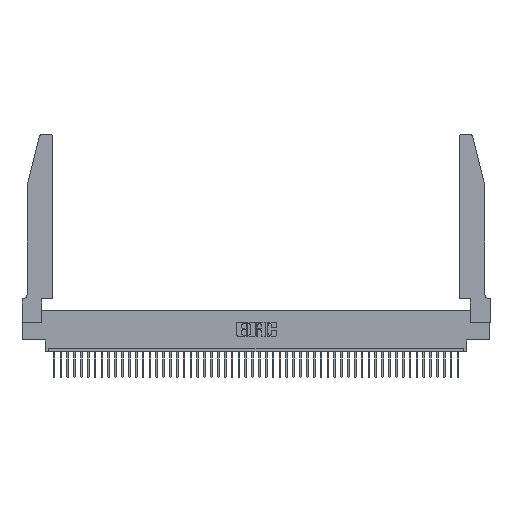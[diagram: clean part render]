
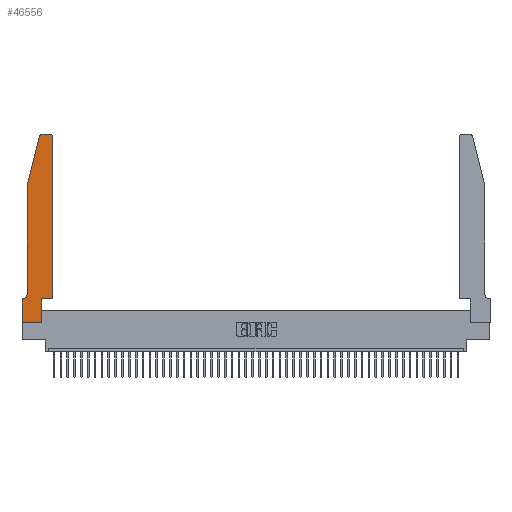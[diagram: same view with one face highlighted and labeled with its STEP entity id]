
A CAD part, top view. The second image highlights one B-rep face of the part: STEP entity #46556.
In plain terms, the highlighted planar face has unit normal (0, 0, 1).
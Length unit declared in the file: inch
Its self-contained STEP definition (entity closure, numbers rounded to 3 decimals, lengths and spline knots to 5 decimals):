
#683 = DIRECTION ( 'NONE',  ( 0., 1., 0. ) ) ;
#1280 = EDGE_LOOP ( 'NONE', ( #1739, #37646, #26872, #36971, #42703, #25595, #14816, #1479, #3994, #7555, #30606, #16357 ) ) ;
#1479 = ORIENTED_EDGE ( 'NONE', *, *, #37676, .T. ) ;
#1739 = ORIENTED_EDGE ( 'NONE', *, *, #34927, .T. ) ;
#2262 = LINE ( 'NONE', #24176, #37366 ) ;
#2815 = DIRECTION ( 'NONE',  ( 0., -1., 0. ) ) ;
#2891 = CARTESIAN_POINT ( 'NONE',  ( 0.0755, 0.42, 0.37 ) ) ;
#3130 = DIRECTION ( 'NONE',  ( 1., 0., 0. ) ) ;
#3139 = CARTESIAN_POINT ( 'NONE',  ( 0.0755, 2., 0.37 ) ) ;
#3725 = CARTESIAN_POINT ( 'NONE',  ( 0.25487, 2.72718, 0.37 ) ) ;
#3811 = EDGE_CURVE ( 'NONE', #37663, #9982, #31243, .T. ) ;
#3994 = ORIENTED_EDGE ( 'NONE', *, *, #32606, .T. ) ;
#4002 = CARTESIAN_POINT ( 'NONE',  ( 0.0055, 0.35, 0.37 ) ) ;
#4797 = VECTOR ( 'NONE', #9925, 39.37008 ) ;
#5273 = LINE ( 'NONE', #45043, #19057 ) ;
#5633 = CARTESIAN_POINT ( 'NONE',  ( 0.4505, 0.35, 0.37 ) ) ;
#5794 = LINE ( 'NONE', #20876, #12665 ) ;
#5851 = EDGE_CURVE ( 'NONE', #29223, #14498, #2262, .T. ) ;
#6450 = VERTEX_POINT ( 'NONE', #15309 ) ;
#7297 = VERTEX_POINT ( 'NONE', #3725 ) ;
#7555 = ORIENTED_EDGE ( 'NONE', *, *, #16457, .T. ) ;
#7649 = VERTEX_POINT ( 'NONE', #30393 ) ;
#8221 = EDGE_CURVE ( 'NONE', #26927, #13217, #12668, .T. ) ;
#8306 = DIRECTION ( 'NONE',  ( 0., 0., 1. ) ) ;
#8960 = CARTESIAN_POINT ( 'NONE',  ( 0.0755, 2., 0.37 ) ) ;
#9444 = VECTOR ( 'NONE', #21039, 39.37008 ) ;
#9925 = DIRECTION ( 'NONE',  ( -0.239, -0.971, 0. ) ) ;
#9982 = VERTEX_POINT ( 'NONE', #30535 ) ;
#11241 = FACE_OUTER_BOUND ( 'NONE', #1280, .T. ) ;
#12665 = VECTOR ( 'NONE', #46744, 39.37008 ) ;
#12668 = LINE ( 'NONE', #3139, #46632 ) ;
#12776 = CARTESIAN_POINT ( 'NONE',  ( 0.4505, 0.35, 0.37 ) ) ;
#13217 = VERTEX_POINT ( 'NONE', #2891 ) ;
#14498 = VERTEX_POINT ( 'NONE', #45339 ) ;
#14816 = ORIENTED_EDGE ( 'NONE', *, *, #40210, .T. ) ;
#15309 = CARTESIAN_POINT ( 'NONE',  ( 0.2865, 0.35, 0.37 ) ) ;
#15660 = DIRECTION ( 'NONE',  ( 0., -1., 0. ) ) ;
#16357 = ORIENTED_EDGE ( 'NONE', *, *, #33684, .T. ) ;
#16457 = EDGE_CURVE ( 'NONE', #6450, #37663, #5794, .T. ) ;
#17316 = CARTESIAN_POINT ( 'NONE',  ( 0.0755, 2., 0.37 ) ) ;
#18420 = DIRECTION ( 'NONE',  ( 1., 0., 0. ) ) ;
#18593 = CARTESIAN_POINT ( 'NONE',  ( 0.2865, 0., 0.37 ) ) ;
#19057 = VECTOR ( 'NONE', #683, 39.37008 ) ;
#19262 = LINE ( 'NONE', #46527, #32524 ) ;
#19546 = VERTEX_POINT ( 'NONE', #18593 ) ;
#19833 = DIRECTION ( 'NONE',  ( -1., 0., 0. ) ) ;
#20710 = VERTEX_POINT ( 'NONE', #25222 ) ;
#20876 = CARTESIAN_POINT ( 'NONE',  ( 0.4505, 0.35, 0.37 ) ) ;
#21039 = DIRECTION ( 'NONE',  ( -1., 0., 0. ) ) ;
#22398 = AXIS2_PLACEMENT_3D ( 'NONE', #28205, #28688, #3130 ) ;
#22547 = LINE ( 'NONE', #17316, #4797 ) ;
#23108 = LINE ( 'NONE', #44593, #45009 ) ;
#23530 = CIRCLE ( 'NONE', #43765, 0.03 ) ;
#24176 = CARTESIAN_POINT ( 'NONE',  ( 0.0755, 0.35, 0.37 ) ) ;
#25222 = CARTESIAN_POINT ( 'NONE',  ( 0., 0., 0.37 ) ) ;
#25595 = ORIENTED_EDGE ( 'NONE', *, *, #5851, .T. ) ;
#25815 = CARTESIAN_POINT ( 'NONE',  ( 0.4205, 2.72, 0.37 ) ) ;
#26767 = CARTESIAN_POINT ( 'NONE',  ( 0.284, 2.72, 0.37 ) ) ;
#26872 = ORIENTED_EDGE ( 'NONE', *, *, #35549, .T. ) ;
#26927 = VERTEX_POINT ( 'NONE', #8960 ) ;
#28205 = CARTESIAN_POINT ( 'NONE',  ( 0., 0.35, 0.37 ) ) ;
#28688 = DIRECTION ( 'NONE',  ( 0., 0., 1. ) ) ;
#28743 = DIRECTION ( 'NONE',  ( 0., 0., 1. ) ) ;
#29223 = VERTEX_POINT ( 'NONE', #4002 ) ;
#30393 = CARTESIAN_POINT ( 'NONE',  ( 0.4205, 2.75, 0.37 ) ) ;
#30535 = CARTESIAN_POINT ( 'NONE',  ( 0.4505, 2.72, 0.37 ) ) ;
#30606 = ORIENTED_EDGE ( 'NONE', *, *, #3811, .T. ) ;
#30744 = VERTEX_POINT ( 'NONE', #34599 ) ;
#31243 = LINE ( 'NONE', #5633, #45607 ) ;
#31320 = LINE ( 'NONE', #38427, #9444 ) ;
#32524 = VECTOR ( 'NONE', #38518, 39.37008 ) ;
#32606 = EDGE_CURVE ( 'NONE', #19546, #6450, #5273, .T. ) ;
#33684 = EDGE_CURVE ( 'NONE', #9982, #7649, #23530, .T. ) ;
#34569 = DIRECTION ( 'NONE',  ( 0., 1., 0. ) ) ;
#34599 = CARTESIAN_POINT ( 'NONE',  ( 0.284, 2.75, 0.37 ) ) ;
#34927 = EDGE_CURVE ( 'NONE', #7649, #30744, #31320, .T. ) ;
#35549 = EDGE_CURVE ( 'NONE', #7297, #26927, #22547, .T. ) ;
#35921 = EDGE_CURVE ( 'NONE', #13217, #29223, #45556, .T. ) ;
#36971 = ORIENTED_EDGE ( 'NONE', *, *, #8221, .T. ) ;
#37366 = VECTOR ( 'NONE', #40913, 39.37008 ) ;
#37646 = ORIENTED_EDGE ( 'NONE', *, *, #46249, .T. ) ;
#37663 = VERTEX_POINT ( 'NONE', #12776 ) ;
#37676 = EDGE_CURVE ( 'NONE', #20710, #19546, #19262, .T. ) ;
#37868 = DIRECTION ( 'NONE',  ( 0., 0., -1. ) ) ;
#38427 = CARTESIAN_POINT ( 'NONE',  ( 0.2605, 2.75, 0.37 ) ) ;
#38518 = DIRECTION ( 'NONE',  ( 1., 0., 0. ) ) ;
#40210 = EDGE_CURVE ( 'NONE', #14498, #20710, #23108, .T. ) ;
#40913 = DIRECTION ( 'NONE',  ( -1., 0., 0. ) ) ;
#41208 = CIRCLE ( 'NONE', #43070, 0.03 ) ;
#41726 = CARTESIAN_POINT ( 'NONE',  ( 0.0055, 0.42, 0.37 ) ) ;
#42297 = AXIS2_PLACEMENT_3D ( 'NONE', #41726, #37868, #19833 ) ;
#42703 = ORIENTED_EDGE ( 'NONE', *, *, #35921, .T. ) ;
#43070 = AXIS2_PLACEMENT_3D ( 'NONE', #26767, #8306, #45577 ) ;
#43765 = AXIS2_PLACEMENT_3D ( 'NONE', #25815, #28743, #18420 ) ;
#44593 = CARTESIAN_POINT ( 'NONE',  ( 0., 0., 0.37 ) ) ;
#45009 = VECTOR ( 'NONE', #15660, 39.37008 ) ;
#45043 = CARTESIAN_POINT ( 'NONE',  ( 0.2865, 0.35, 0.37 ) ) ;
#45339 = CARTESIAN_POINT ( 'NONE',  ( 0., 0.35, 0.37 ) ) ;
#45556 = CIRCLE ( 'NONE', #42297, 0.07 ) ;
#45577 = DIRECTION ( 'NONE',  ( 1., 0., 0. ) ) ;
#45607 = VECTOR ( 'NONE', #34569, 39.37008 ) ;
#46249 = EDGE_CURVE ( 'NONE', #30744, #7297, #41208, .T. ) ;
#46513 = PLANE ( 'NONE',  #22398 ) ;
#46527 = CARTESIAN_POINT ( 'NONE',  ( 0., 0., 0.37 ) ) ;
#46556 = ADVANCED_FACE ( 'NONE', ( #11241 ), #46513, .T. ) ;
#46632 = VECTOR ( 'NONE', #2815, 39.37008 ) ;
#46744 = DIRECTION ( 'NONE',  ( 1., 0., 0. ) ) ;
